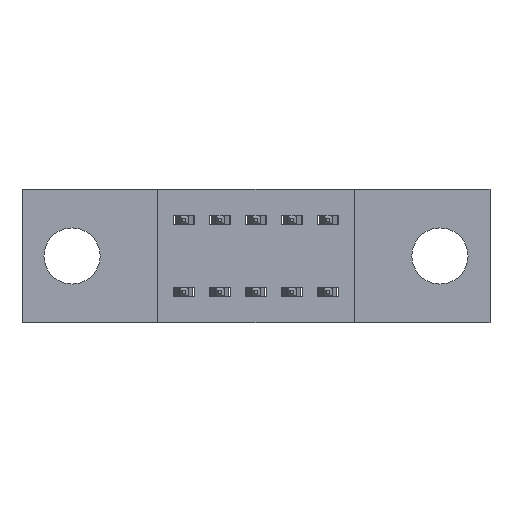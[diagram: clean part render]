
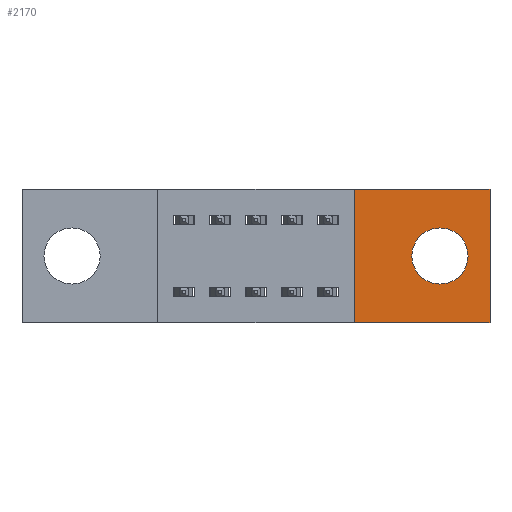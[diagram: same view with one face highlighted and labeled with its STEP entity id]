
A CAD part, front view. The second image highlights one B-rep face of the part: STEP entity #2170.
In plain terms, the highlighted planar face has unit normal (0, -1, 0).
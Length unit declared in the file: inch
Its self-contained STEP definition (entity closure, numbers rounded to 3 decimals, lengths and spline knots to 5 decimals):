
#254 = VERTEX_POINT ( 'NONE', #7013 ) ;
#287 = AXIS2_PLACEMENT_3D ( 'NONE', #5165, #7347, #7328 ) ;
#589 = FACE_BOUND ( 'NONE', #5767, .T. ) ;
#669 = CARTESIAN_POINT ( 'NONE',  ( 0.923, 0., -0.37 ) ) ;
#824 = LINE ( 'NONE', #6172, #7153 ) ;
#1153 = CARTESIAN_POINT ( 'NONE',  ( 1.161, 0., -0.263 ) ) ;
#1370 = VERTEX_POINT ( 'NONE', #669 ) ;
#1491 = ORIENTED_EDGE ( 'NONE', *, *, #4290, .F. ) ;
#1555 = ORIENTED_EDGE ( 'NONE', *, *, #4240, .F. ) ;
#1902 = ORIENTED_EDGE ( 'NONE', *, *, #4130, .T. ) ;
#2005 = VERTEX_POINT ( 'NONE', #7514 ) ;
#2170 = ADVANCED_FACE ( 'NONE', ( #589, #6974 ), #6944, .T. ) ;
#2715 = CARTESIAN_POINT ( 'NONE',  ( 0., 0., 0. ) ) ;
#2837 = CARTESIAN_POINT ( 'NONE',  ( 1.161, 0., -0.107 ) ) ;
#3255 = VERTEX_POINT ( 'NONE', #2837 ) ;
#3278 = VERTEX_POINT ( 'NONE', #1153 ) ;
#3461 = VERTEX_POINT ( 'NONE', #5231 ) ;
#3495 = EDGE_CURVE ( 'NONE', #3278, #3255, #6232, .T. ) ;
#3662 = CIRCLE ( 'NONE', #5076, 0.078 ) ;
#4130 = EDGE_CURVE ( 'NONE', #3255, #3278, #3662, .T. ) ;
#4240 = EDGE_CURVE ( 'NONE', #1370, #3461, #5792, .T. ) ;
#4290 = EDGE_CURVE ( 'NONE', #2005, #1370, #5434, .T. ) ;
#4429 = EDGE_CURVE ( 'NONE', #254, #2005, #824, .T. ) ;
#4526 = LINE ( 'NONE', #2715, #7297 ) ;
#4597 = ORIENTED_EDGE ( 'NONE', *, *, #3495, .T. ) ;
#5061 = ORIENTED_EDGE ( 'NONE', *, *, #7052, .F. ) ;
#5076 = AXIS2_PLACEMENT_3D ( 'NONE', #7872, #7863, #7857 ) ;
#5165 = CARTESIAN_POINT ( 'NONE',  ( 0., 0., -0.37 ) ) ;
#5231 = CARTESIAN_POINT ( 'NONE',  ( 0.923, 0., 0. ) ) ;
#5434 = LINE ( 'NONE', #6794, #6721 ) ;
#5453 = ORIENTED_EDGE ( 'NONE', *, *, #4429, .F. ) ;
#5622 = VECTOR ( 'NONE', #7212, 39.37008 ) ;
#5763 = DIRECTION ( 'NONE',  ( 1., 0., 0. ) ) ;
#5767 = EDGE_LOOP ( 'NONE', ( #1902, #4597 ) ) ;
#5792 = LINE ( 'NONE', #7558, #5622 ) ;
#6062 = DIRECTION ( 'NONE',  ( 0., 0., -1. ) ) ;
#6172 = CARTESIAN_POINT ( 'NONE',  ( 1.3, 0., 0. ) ) ;
#6232 = CIRCLE ( 'NONE', #6324, 0.078 ) ;
#6324 = AXIS2_PLACEMENT_3D ( 'NONE', #7578, #7690, #7712 ) ;
#6721 = VECTOR ( 'NONE', #6782, 39.37008 ) ;
#6782 = DIRECTION ( 'NONE',  ( -1., 0., 0. ) ) ;
#6794 = CARTESIAN_POINT ( 'NONE',  ( 0., 0., -0.37 ) ) ;
#6944 = PLANE ( 'NONE',  #287 ) ;
#6974 = FACE_OUTER_BOUND ( 'NONE', #7197, .T. ) ;
#7013 = CARTESIAN_POINT ( 'NONE',  ( 1.3, 0., 0. ) ) ;
#7052 = EDGE_CURVE ( 'NONE', #3461, #254, #4526, .T. ) ;
#7153 = VECTOR ( 'NONE', #6062, 39.37008 ) ;
#7197 = EDGE_LOOP ( 'NONE', ( #1555, #1491, #5453, #5061 ) ) ;
#7212 = DIRECTION ( 'NONE',  ( 0., 0., 1. ) ) ;
#7297 = VECTOR ( 'NONE', #5763, 39.37008 ) ;
#7328 = DIRECTION ( 'NONE',  ( 0., 0., -1. ) ) ;
#7347 = DIRECTION ( 'NONE',  ( 0., -1., 0. ) ) ;
#7514 = CARTESIAN_POINT ( 'NONE',  ( 1.3, 0., -0.37 ) ) ;
#7558 = CARTESIAN_POINT ( 'NONE',  ( 0.923, 0., -0.37 ) ) ;
#7578 = CARTESIAN_POINT ( 'NONE',  ( 1.161, 0., -0.185 ) ) ;
#7690 = DIRECTION ( 'NONE',  ( 0., 1., 0. ) ) ;
#7712 = DIRECTION ( 'NONE',  ( 0., 0., -1. ) ) ;
#7857 = DIRECTION ( 'NONE',  ( 0., 0., -1. ) ) ;
#7863 = DIRECTION ( 'NONE',  ( 0., 1., 0. ) ) ;
#7872 = CARTESIAN_POINT ( 'NONE',  ( 1.161, 0., -0.185 ) ) ;
